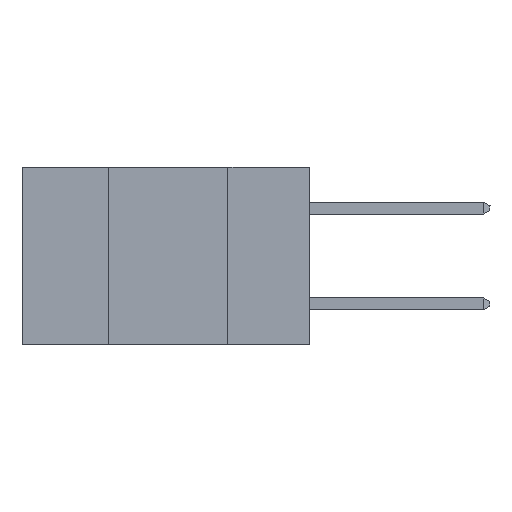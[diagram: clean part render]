
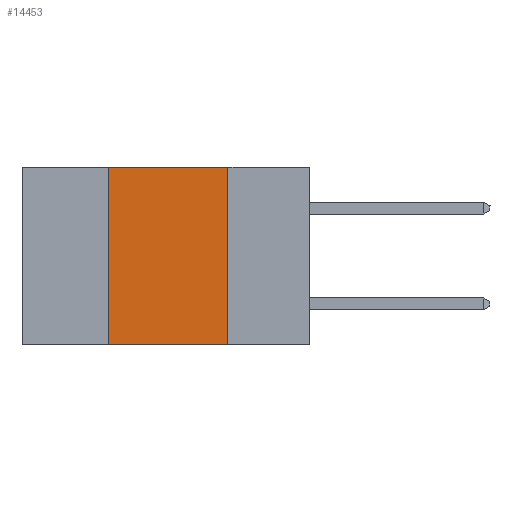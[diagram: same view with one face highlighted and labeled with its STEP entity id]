
A CAD part, left-side view. The second image highlights one B-rep face of the part: STEP entity #14453.
In plain terms, the highlighted planar face has unit normal (-1, 0, 0).
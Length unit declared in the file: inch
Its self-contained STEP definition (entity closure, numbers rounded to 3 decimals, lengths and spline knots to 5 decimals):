
#412 = VECTOR ( 'NONE', #8148, 39.37008 ) ;
#855 = VERTEX_POINT ( 'NONE', #21536 ) ;
#898 = ORIENTED_EDGE ( 'NONE', *, *, #14792, .F. ) ;
#1307 = EDGE_CURVE ( 'NONE', #855, #20262, #11035, .T. ) ;
#2464 = FACE_OUTER_BOUND ( 'NONE', #22480, .T. ) ;
#3429 = VERTEX_POINT ( 'NONE', #4668 ) ;
#4044 = LINE ( 'NONE', #10230, #20966 ) ;
#4668 = CARTESIAN_POINT ( 'NONE',  ( 0., 0.42, -0.37 ) ) ;
#6277 = CARTESIAN_POINT ( 'NONE',  ( 0., 0.17, -0.37 ) ) ;
#8148 = DIRECTION ( 'NONE',  ( 0., -1., 0. ) ) ;
#8404 = EDGE_CURVE ( 'NONE', #3429, #14318, #4044, .T. ) ;
#9941 = PLANE ( 'NONE',  #14030 ) ;
#10230 = CARTESIAN_POINT ( 'NONE',  ( 0., 0.42, 0. ) ) ;
#11035 = LINE ( 'NONE', #19540, #19184 ) ;
#11688 = DIRECTION ( 'NONE',  ( 0., 0., -1. ) ) ;
#11768 = CARTESIAN_POINT ( 'NONE',  ( 0., 0.6, 0. ) ) ;
#12198 = DIRECTION ( 'NONE',  ( 0., 0., 1. ) ) ;
#13406 = CARTESIAN_POINT ( 'NONE',  ( 0., 0.6, -0.37 ) ) ;
#14030 = AXIS2_PLACEMENT_3D ( 'NONE', #11768, #22126, #11688 ) ;
#14318 = VERTEX_POINT ( 'NONE', #21587 ) ;
#14453 = ADVANCED_FACE ( 'NONE', ( #2464 ), #9941, .F. ) ;
#14792 = EDGE_CURVE ( 'NONE', #14318, #855, #19076, .T. ) ;
#14872 = LINE ( 'NONE', #13406, #412 ) ;
#16325 = DIRECTION ( 'NONE',  ( 0., 0., -1. ) ) ;
#17758 = ORIENTED_EDGE ( 'NONE', *, *, #8404, .F. ) ;
#17886 = CARTESIAN_POINT ( 'NONE',  ( 0., 0.6, 0. ) ) ;
#19076 = LINE ( 'NONE', #17886, #19623 ) ;
#19184 = VECTOR ( 'NONE', #16325, 39.37008 ) ;
#19238 = ORIENTED_EDGE ( 'NONE', *, *, #1307, .F. ) ;
#19540 = CARTESIAN_POINT ( 'NONE',  ( 0., 0.17, 0. ) ) ;
#19543 = DIRECTION ( 'NONE',  ( 0., -1., 0. ) ) ;
#19623 = VECTOR ( 'NONE', #19543, 39.37008 ) ;
#20095 = ORIENTED_EDGE ( 'NONE', *, *, #21573, .T. ) ;
#20262 = VERTEX_POINT ( 'NONE', #6277 ) ;
#20966 = VECTOR ( 'NONE', #12198, 39.37008 ) ;
#21536 = CARTESIAN_POINT ( 'NONE',  ( 0., 0.17, 0. ) ) ;
#21573 = EDGE_CURVE ( 'NONE', #3429, #20262, #14872, .T. ) ;
#21587 = CARTESIAN_POINT ( 'NONE',  ( 0., 0.42, 0. ) ) ;
#22126 = DIRECTION ( 'NONE',  ( 1., 0., 0. ) ) ;
#22480 = EDGE_LOOP ( 'NONE', ( #19238, #898, #17758, #20095 ) ) ;
